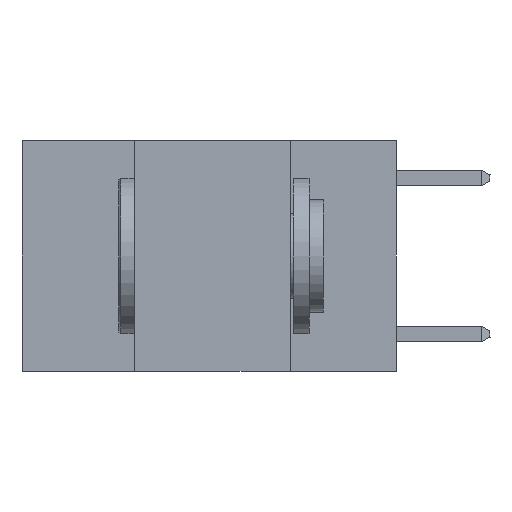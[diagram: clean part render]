
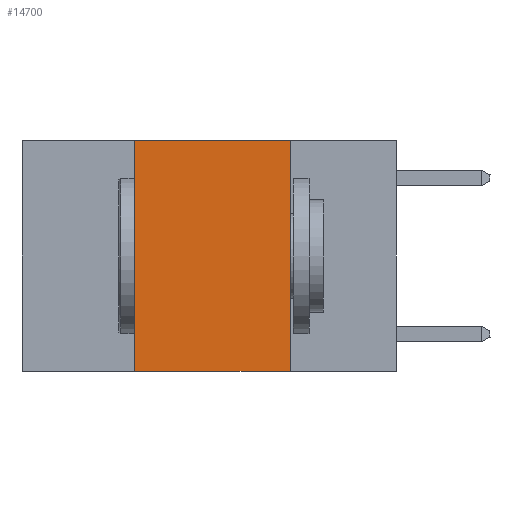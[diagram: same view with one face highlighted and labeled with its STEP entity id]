
A CAD part, left-side view. The second image highlights one B-rep face of the part: STEP entity #14700.
In plain terms, the highlighted planar face has unit normal (-1, 0, 0).
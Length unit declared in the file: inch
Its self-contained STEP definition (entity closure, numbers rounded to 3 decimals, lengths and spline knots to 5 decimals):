
#964 = DIRECTION ( 'NONE',  ( 0., -1., 0. ) ) ;
#1080 = VECTOR ( 'NONE', #10321, 39.37008 ) ;
#1084 = LINE ( 'NONE', #4692, #2941 ) ;
#1819 = VERTEX_POINT ( 'NONE', #3727 ) ;
#2941 = VECTOR ( 'NONE', #964, 39.37008 ) ;
#3022 = DIRECTION ( 'NONE',  ( 0., 0., -1. ) ) ;
#3516 = EDGE_CURVE ( 'NONE', #1819, #4651, #1084, .T. ) ;
#3727 = CARTESIAN_POINT ( 'NONE',  ( 0., 0.42, 0. ) ) ;
#4486 = ORIENTED_EDGE ( 'NONE', *, *, #17844, .F. ) ;
#4651 = VERTEX_POINT ( 'NONE', #15790 ) ;
#4692 = CARTESIAN_POINT ( 'NONE',  ( 0., 0.6, 0. ) ) ;
#4942 = EDGE_LOOP ( 'NONE', ( #5476, #16051, #4486, #9483 ) ) ;
#5004 = CARTESIAN_POINT ( 'NONE',  ( 0., 0.6, -0.37 ) ) ;
#5476 = ORIENTED_EDGE ( 'NONE', *, *, #8230, .F. ) ;
#6041 = VECTOR ( 'NONE', #9685, 39.37008 ) ;
#6518 = CARTESIAN_POINT ( 'NONE',  ( 0., 0.6, 0. ) ) ;
#7137 = CARTESIAN_POINT ( 'NONE',  ( 0., 0.17, -0.37 ) ) ;
#7144 = AXIS2_PLACEMENT_3D ( 'NONE', #6518, #13696, #3022 ) ;
#8230 = EDGE_CURVE ( 'NONE', #4651, #10878, #11751, .T. ) ;
#9483 = ORIENTED_EDGE ( 'NONE', *, *, #22213, .T. ) ;
#9558 = CARTESIAN_POINT ( 'NONE',  ( 0., 0.42, 0. ) ) ;
#9685 = DIRECTION ( 'NONE',  ( 0., 0., -1. ) ) ;
#10321 = DIRECTION ( 'NONE',  ( 0., -1., 0. ) ) ;
#10878 = VERTEX_POINT ( 'NONE', #7137 ) ;
#11405 = CARTESIAN_POINT ( 'NONE',  ( 0., 0.17, 0. ) ) ;
#11751 = LINE ( 'NONE', #11405, #6041 ) ;
#12167 = CARTESIAN_POINT ( 'NONE',  ( 0., 0.42, -0.37 ) ) ;
#13495 = LINE ( 'NONE', #9558, #17102 ) ;
#13696 = DIRECTION ( 'NONE',  ( 1., 0., 0. ) ) ;
#13814 = LINE ( 'NONE', #5004, #1080 ) ;
#14700 = ADVANCED_FACE ( 'NONE', ( #15317 ), #22429, .F. ) ;
#15317 = FACE_OUTER_BOUND ( 'NONE', #4942, .T. ) ;
#15790 = CARTESIAN_POINT ( 'NONE',  ( 0., 0.17, 0. ) ) ;
#16051 = ORIENTED_EDGE ( 'NONE', *, *, #3516, .F. ) ;
#17102 = VECTOR ( 'NONE', #22689, 39.37008 ) ;
#17844 = EDGE_CURVE ( 'NONE', #22144, #1819, #13495, .T. ) ;
#22144 = VERTEX_POINT ( 'NONE', #12167 ) ;
#22213 = EDGE_CURVE ( 'NONE', #22144, #10878, #13814, .T. ) ;
#22429 = PLANE ( 'NONE',  #7144 ) ;
#22689 = DIRECTION ( 'NONE',  ( 0., 0., 1. ) ) ;
